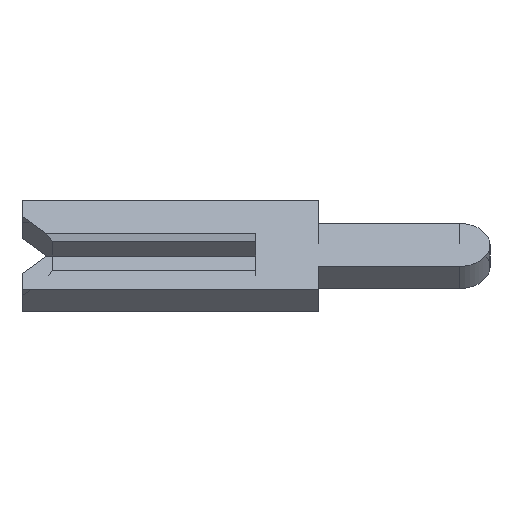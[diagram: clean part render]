
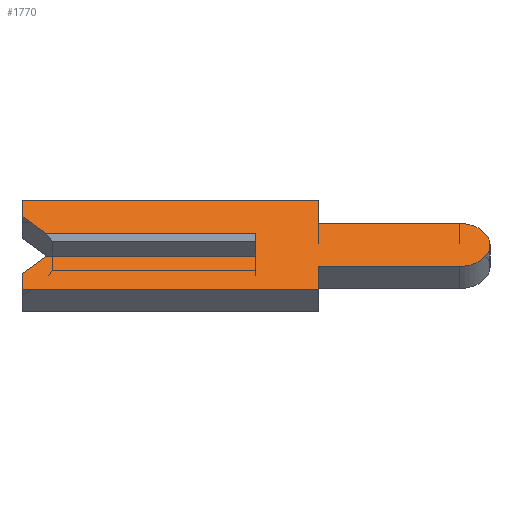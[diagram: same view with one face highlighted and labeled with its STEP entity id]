
A CAD part, left-side view. The second image highlights one B-rep face of the part: STEP entity #1770.
In plain terms, the highlighted face is planar.
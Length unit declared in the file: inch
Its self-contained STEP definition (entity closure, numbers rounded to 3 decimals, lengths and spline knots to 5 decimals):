
#8 = VECTOR ( 'NONE', #230, 39.37008 ) ;
#11 = ORIENTED_EDGE ( 'NONE', *, *, #183, .F. ) ;
#26 = CARTESIAN_POINT ( 'NONE',  ( -0.01, -0.04, -0.0195 ) ) ;
#29 = CARTESIAN_POINT ( 'NONE',  ( -0.01, -0.04, 0.04 ) ) ;
#39 = VERTEX_POINT ( 'NONE', #1023 ) ;
#57 = CARTESIAN_POINT ( 'NONE',  ( -0.01, 0.1305, -0.0065 ) ) ;
#75 = CARTESIAN_POINT ( 'NONE',  ( -0.01, -0.1305, -0.0195 ) ) ;
#79 = LINE ( 'NONE', #1533, #953 ) ;
#82 = CARTESIAN_POINT ( 'NONE',  ( -0.01, -0.1305, -0.01 ) ) ;
#83 = VERTEX_POINT ( 'NONE', #731 ) ;
#114 = EDGE_CURVE ( 'NONE', #83, #1723, #1345, .T. ) ;
#141 = CARTESIAN_POINT ( 'NONE',  ( -0.01, 0.15, 0.01 ) ) ;
#147 = CARTESIAN_POINT ( 'NONE',  ( -0.01, 0., 0.0065 ) ) ;
#152 = DIRECTION ( 'NONE',  ( 0., 0., 1. ) ) ;
#160 = DIRECTION ( 'NONE',  ( 0., 0., 1. ) ) ;
#169 = DIRECTION ( 'NONE',  ( 0., -1., 0. ) ) ;
#173 = VECTOR ( 'NONE', #1110, 39.37008 ) ;
#183 = EDGE_CURVE ( 'NONE', #786, #1723, #807, .T. ) ;
#195 = CARTESIAN_POINT ( 'NONE',  ( -0.01, -0.04, -0.0195 ) ) ;
#222 = CARTESIAN_POINT ( 'NONE',  ( -0.01, 0.1305, 0.0065 ) ) ;
#230 = DIRECTION ( 'NONE',  ( 0., 0.707, 0.707 ) ) ;
#265 = LINE ( 'NONE', #1411, #173 ) ;
#302 = CARTESIAN_POINT ( 'NONE',  ( -0.01, 0.15, 0.026 ) ) ;
#313 = ORIENTED_EDGE ( 'NONE', *, *, #1774, .F. ) ;
#366 = DIRECTION ( 'NONE',  ( 1., 0., 0. ) ) ;
#374 = PLANE ( 'NONE',  #1670 ) ;
#400 = ORIENTED_EDGE ( 'NONE', *, *, #841, .F. ) ;
#445 = VERTEX_POINT ( 'NONE', #29 ) ;
#484 = DIRECTION ( 'NONE',  ( 0., 1., 0. ) ) ;
#497 = VERTEX_POINT ( 'NONE', #1359 ) ;
#507 = DIRECTION ( 'NONE',  ( 0., 0., -1. ) ) ;
#510 = CARTESIAN_POINT ( 'NONE',  ( -0.01, -0.04, 0.0195 ) ) ;
#523 = CARTESIAN_POINT ( 'NONE',  ( -0.01, 0.15, 0.026 ) ) ;
#533 = VECTOR ( 'NONE', #160, 39.37008 ) ;
#545 = EDGE_CURVE ( 'NONE', #742, #497, #856, .T. ) ;
#568 = EDGE_CURVE ( 'NONE', #445, #864, #79, .T. ) ;
#610 = DIRECTION ( 'NONE',  ( 0., 0., -1. ) ) ;
#622 = LINE ( 'NONE', #1396, #897 ) ;
#623 = VECTOR ( 'NONE', #1667, 39.37008 ) ;
#635 = DIRECTION ( 'NONE',  ( 0., 0., -1. ) ) ;
#637 = DIRECTION ( 'NONE',  ( 0., 0., -1. ) ) ;
#645 = VECTOR ( 'NONE', #610, 39.37008 ) ;
#646 = DIRECTION ( 'NONE',  ( 0., -1., 0. ) ) ;
#669 = LINE ( 'NONE', #1524, #645 ) ;
#694 = LINE ( 'NONE', #82, #1273 ) ;
#706 = EDGE_CURVE ( 'NONE', #39, #445, #265, .T. ) ;
#720 = VECTOR ( 'NONE', #169, 39.37008 ) ;
#731 = CARTESIAN_POINT ( 'NONE',  ( -0.01, 0.134, 0.01 ) ) ;
#739 = VERTEX_POINT ( 'NONE', #1708 ) ;
#742 = VERTEX_POINT ( 'NONE', #1688 ) ;
#743 = VERTEX_POINT ( 'NONE', #946 ) ;
#775 = CARTESIAN_POINT ( 'NONE',  ( -0.01, 0.15, -0.026 ) ) ;
#782 = ORIENTED_EDGE ( 'NONE', *, *, #114, .T. ) ;
#786 = VERTEX_POINT ( 'NONE', #814 ) ;
#794 = CARTESIAN_POINT ( 'NONE',  ( -0.01, -0.04, 0.0195 ) ) ;
#795 = CARTESIAN_POINT ( 'NONE',  ( -0.01, 0., 0.01 ) ) ;
#800 = CARTESIAN_POINT ( 'NONE',  ( -0.01, -0.1305, 0. ) ) ;
#807 = LINE ( 'NONE', #147, #533 ) ;
#814 = CARTESIAN_POINT ( 'NONE',  ( -0.01, 0., -0.01 ) ) ;
#841 = EDGE_CURVE ( 'NONE', #864, #743, #1251, .T. ) ;
#856 = LINE ( 'NONE', #775, #623 ) ;
#864 = VERTEX_POINT ( 'NONE', #794 ) ;
#897 = VECTOR ( 'NONE', #1695, 39.37008 ) ;
#901 = ORIENTED_EDGE ( 'NONE', *, *, #545, .F. ) ;
#926 = DIRECTION ( 'NONE',  ( 0., -0.707, 0.707 ) ) ;
#946 = CARTESIAN_POINT ( 'NONE',  ( -0.01, -0.1305, 0.0195 ) ) ;
#953 = VECTOR ( 'NONE', #637, 39.37008 ) ;
#956 = ORIENTED_EDGE ( 'NONE', *, *, #1675, .F. ) ;
#1018 = LINE ( 'NONE', #57, #1462 ) ;
#1020 = ORIENTED_EDGE ( 'NONE', *, *, #1108, .F. ) ;
#1023 = CARTESIAN_POINT ( 'NONE',  ( -0.01, 0.15, 0.04 ) ) ;
#1061 = CARTESIAN_POINT ( 'NONE',  ( -0.01, -0.04, -0.04 ) ) ;
#1102 = ORIENTED_EDGE ( 'NONE', *, *, #1702, .F. ) ;
#1108 = EDGE_CURVE ( 'NONE', #1764, #39, #1293, .T. ) ;
#1110 = DIRECTION ( 'NONE',  ( 0., -1., 0. ) ) ;
#1116 = VERTEX_POINT ( 'NONE', #26 ) ;
#1156 = LINE ( 'NONE', #195, #1854 ) ;
#1181 = VECTOR ( 'NONE', #152, 39.37008 ) ;
#1220 = DIRECTION ( 'NONE',  ( 1., 0., 0. ) ) ;
#1251 = LINE ( 'NONE', #510, #1412 ) ;
#1260 = ORIENTED_EDGE ( 'NONE', *, *, #568, .F. ) ;
#1266 = AXIS2_PLACEMENT_3D ( 'NONE', #1516, #1220, #635 ) ;
#1273 = VECTOR ( 'NONE', #646, 39.37008 ) ;
#1293 = LINE ( 'NONE', #302, #1181 ) ;
#1323 = VERTEX_POINT ( 'NONE', #1061 ) ;
#1342 = FACE_OUTER_BOUND ( 'NONE', #1721, .T. ) ;
#1345 = LINE ( 'NONE', #141, #720 ) ;
#1359 = CARTESIAN_POINT ( 'NONE',  ( -0.01, 0.15, -0.026 ) ) ;
#1365 = EDGE_CURVE ( 'NONE', #1116, #1323, #669, .T. ) ;
#1370 = ORIENTED_EDGE ( 'NONE', *, *, #1501, .F. ) ;
#1396 = CARTESIAN_POINT ( 'NONE',  ( -0.01, 0.15, -0.04 ) ) ;
#1411 = CARTESIAN_POINT ( 'NONE',  ( -0.01, 0.15, 0.04 ) ) ;
#1412 = VECTOR ( 'NONE', #1852, 39.37008 ) ;
#1434 = EDGE_CURVE ( 'NONE', #743, #1676, #1656, .T. ) ;
#1445 = ORIENTED_EDGE ( 'NONE', *, *, #1365, .F. ) ;
#1462 = VECTOR ( 'NONE', #926, 39.37008 ) ;
#1475 = EDGE_CURVE ( 'NONE', #1676, #1116, #1156, .T. ) ;
#1501 = EDGE_CURVE ( 'NONE', #497, #739, #1018, .T. ) ;
#1516 = CARTESIAN_POINT ( 'NONE',  ( -0.01, -0.1305, 0. ) ) ;
#1524 = CARTESIAN_POINT ( 'NONE',  ( -0.01, -0.04, -0.04 ) ) ;
#1533 = CARTESIAN_POINT ( 'NONE',  ( -0.01, -0.04, 0.04 ) ) ;
#1544 = ORIENTED_EDGE ( 'NONE', *, *, #1475, .F. ) ;
#1656 = CIRCLE ( 'NONE', #1266, 0.0195 ) ;
#1667 = DIRECTION ( 'NONE',  ( 0., 0., 1. ) ) ;
#1670 = AXIS2_PLACEMENT_3D ( 'NONE', #800, #366, #507 ) ;
#1675 = EDGE_CURVE ( 'NONE', #83, #1764, #1874, .T. ) ;
#1676 = VERTEX_POINT ( 'NONE', #75 ) ;
#1681 = ORIENTED_EDGE ( 'NONE', *, *, #706, .F. ) ;
#1688 = CARTESIAN_POINT ( 'NONE',  ( -0.01, 0.15, -0.04 ) ) ;
#1695 = DIRECTION ( 'NONE',  ( 0., 1., 0. ) ) ;
#1702 = EDGE_CURVE ( 'NONE', #1323, #742, #622, .T. ) ;
#1708 = CARTESIAN_POINT ( 'NONE',  ( -0.01, 0.134, -0.01 ) ) ;
#1721 = EDGE_LOOP ( 'NONE', ( #782, #11, #313, #1370, #901, #1102, #1445, #1544, #1792, #400, #1260, #1681, #1020, #956 ) ) ;
#1723 = VERTEX_POINT ( 'NONE', #795 ) ;
#1764 = VERTEX_POINT ( 'NONE', #523 ) ;
#1770 = ADVANCED_FACE ( 'NONE', ( #1342 ), #374, .F. ) ;
#1774 = EDGE_CURVE ( 'NONE', #739, #786, #694, .T. ) ;
#1792 = ORIENTED_EDGE ( 'NONE', *, *, #1434, .F. ) ;
#1852 = DIRECTION ( 'NONE',  ( 0., -1., 0. ) ) ;
#1854 = VECTOR ( 'NONE', #484, 39.37008 ) ;
#1874 = LINE ( 'NONE', #222, #8 ) ;
